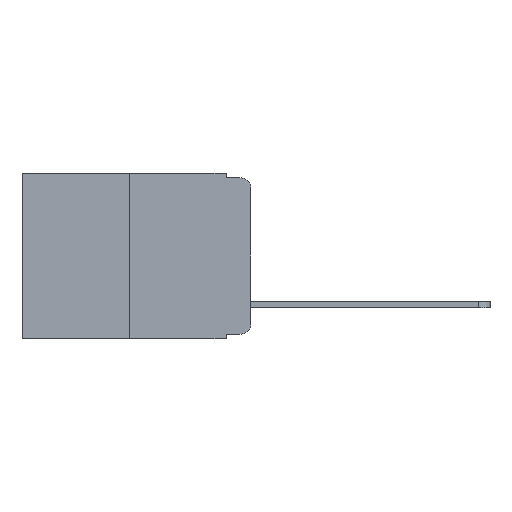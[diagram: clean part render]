
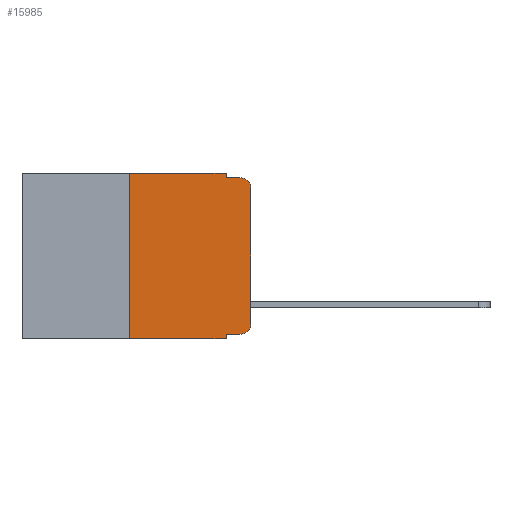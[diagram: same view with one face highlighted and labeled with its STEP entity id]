
A CAD part, left-side view. The second image highlights one B-rep face of the part: STEP entity #15985.
In plain terms, the highlighted planar face has unit normal (-1, 0, 0).
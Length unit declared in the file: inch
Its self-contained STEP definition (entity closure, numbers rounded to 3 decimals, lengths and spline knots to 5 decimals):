
#923 = VERTEX_POINT ( 'NONE', #13143 ) ;
#1006 = VERTEX_POINT ( 'NONE', #2256 ) ;
#1129 = CARTESIAN_POINT ( 'NONE',  ( 0., 0., 0. ) ) ;
#1184 = DIRECTION ( 'NONE',  ( 1., 0., 0. ) ) ;
#1445 = AXIS2_PLACEMENT_3D ( 'NONE', #12316, #3045, #13771 ) ;
#1646 = CARTESIAN_POINT ( 'NONE',  ( 0., 0.02, -0.01 ) ) ;
#1650 = CARTESIAN_POINT ( 'NONE',  ( 0., 0.051, -0.343 ) ) ;
#1653 = CIRCLE ( 'NONE', #1445, 0.02 ) ;
#1670 = CARTESIAN_POINT ( 'NONE',  ( 0., 0.473, -0.343 ) ) ;
#1677 = VERTEX_POINT ( 'NONE', #1650 ) ;
#2256 = CARTESIAN_POINT ( 'NONE',  ( 0., 0., -0.03 ) ) ;
#2742 = CARTESIAN_POINT ( 'NONE',  ( 0., 0.25, 0. ) ) ;
#2957 = LINE ( 'NONE', #1670, #15027 ) ;
#3012 = CARTESIAN_POINT ( 'NONE',  ( 0., 0.051, -0.01 ) ) ;
#3045 = DIRECTION ( 'NONE',  ( -1., 0., 0. ) ) ;
#3402 = DIRECTION ( 'NONE',  ( 0., -1., 0. ) ) ;
#3897 = VECTOR ( 'NONE', #16217, 39.37008 ) ;
#4248 = ORIENTED_EDGE ( 'NONE', *, *, #9250, .F. ) ;
#4501 = VECTOR ( 'NONE', #13741, 39.37008 ) ;
#4790 = ORIENTED_EDGE ( 'NONE', *, *, #9302, .F. ) ;
#4980 = DIRECTION ( 'NONE',  ( 0., 0., -1. ) ) ;
#5019 = CIRCLE ( 'NONE', #13310, 0.02 ) ;
#5287 = ORIENTED_EDGE ( 'NONE', *, *, #7506, .T. ) ;
#5894 = EDGE_CURVE ( 'NONE', #7233, #923, #14680, .T. ) ;
#5924 = CARTESIAN_POINT ( 'NONE',  ( 0., 0.051, -0.01 ) ) ;
#6185 = CARTESIAN_POINT ( 'NONE',  ( 0., 0.25, 0. ) ) ;
#6315 = CARTESIAN_POINT ( 'NONE',  ( 0., 0.051, -0.333 ) ) ;
#6357 = CARTESIAN_POINT ( 'NONE',  ( 0., 0.02, -0.03 ) ) ;
#6660 = VERTEX_POINT ( 'NONE', #11933 ) ;
#6905 = VECTOR ( 'NONE', #14562, 39.37008 ) ;
#7233 = VERTEX_POINT ( 'NONE', #2742 ) ;
#7506 = EDGE_CURVE ( 'NONE', #13405, #1677, #2957, .T. ) ;
#7651 = VECTOR ( 'NONE', #4980, 39.37008 ) ;
#7692 = CARTESIAN_POINT ( 'NONE',  ( 0., 0.051, 0. ) ) ;
#7870 = DIRECTION ( 'NONE',  ( 0., 0., -1. ) ) ;
#8481 = AXIS2_PLACEMENT_3D ( 'NONE', #9200, #1184, #12219 ) ;
#8831 = ORIENTED_EDGE ( 'NONE', *, *, #5894, .F. ) ;
#9151 = DIRECTION ( 'NONE',  ( 0., 0., 1. ) ) ;
#9200 = CARTESIAN_POINT ( 'NONE',  ( 0., 0.473, 0. ) ) ;
#9202 = EDGE_CURVE ( 'NONE', #10691, #1006, #17277, .T. ) ;
#9249 = EDGE_CURVE ( 'NONE', #1006, #10289, #5019, .T. ) ;
#9250 = EDGE_CURVE ( 'NONE', #18162, #10289, #16505, .T. ) ;
#9281 = ORIENTED_EDGE ( 'NONE', *, *, #10593, .F. ) ;
#9302 = EDGE_CURVE ( 'NONE', #923, #18162, #18215, .T. ) ;
#10289 = VERTEX_POINT ( 'NONE', #1646 ) ;
#10583 = EDGE_CURVE ( 'NONE', #13405, #7233, #18950, .T. ) ;
#10593 = EDGE_CURVE ( 'NONE', #14069, #1677, #18170, .T. ) ;
#10640 = EDGE_CURVE ( 'NONE', #14069, #6660, #17005, .T. ) ;
#10641 = EDGE_CURVE ( 'NONE', #6660, #10691, #1653, .T. ) ;
#10691 = VERTEX_POINT ( 'NONE', #12448 ) ;
#11402 = ORIENTED_EDGE ( 'NONE', *, *, #9202, .T. ) ;
#11933 = CARTESIAN_POINT ( 'NONE',  ( 0., 0.02, -0.333 ) ) ;
#12219 = DIRECTION ( 'NONE',  ( 0., 0., -1. ) ) ;
#12316 = CARTESIAN_POINT ( 'NONE',  ( 0., 0.02, -0.313 ) ) ;
#12448 = CARTESIAN_POINT ( 'NONE',  ( 0., 0., -0.313 ) ) ;
#12775 = ORIENTED_EDGE ( 'NONE', *, *, #10583, .F. ) ;
#13143 = CARTESIAN_POINT ( 'NONE',  ( 0., 0.051, 0. ) ) ;
#13244 = ORIENTED_EDGE ( 'NONE', *, *, #10640, .T. ) ;
#13310 = AXIS2_PLACEMENT_3D ( 'NONE', #6357, #16346, #7870 ) ;
#13405 = VERTEX_POINT ( 'NONE', #16231 ) ;
#13569 = VECTOR ( 'NONE', #17552, 39.37008 ) ;
#13741 = DIRECTION ( 'NONE',  ( 0., -1., 0. ) ) ;
#13771 = DIRECTION ( 'NONE',  ( 0., 0., -1. ) ) ;
#13917 = CARTESIAN_POINT ( 'NONE',  ( 0., 0.051, 0. ) ) ;
#14069 = VERTEX_POINT ( 'NONE', #15320 ) ;
#14320 = VECTOR ( 'NONE', #9151, 39.37008 ) ;
#14562 = DIRECTION ( 'NONE',  ( 0., -1., 0. ) ) ;
#14680 = LINE ( 'NONE', #17100, #6905 ) ;
#14898 = VECTOR ( 'NONE', #15004, 39.37008 ) ;
#15004 = DIRECTION ( 'NONE',  ( 0., 0., -1. ) ) ;
#15027 = VECTOR ( 'NONE', #3402, 39.37008 ) ;
#15151 = ORIENTED_EDGE ( 'NONE', *, *, #9249, .T. ) ;
#15320 = CARTESIAN_POINT ( 'NONE',  ( 0., 0.051, -0.333 ) ) ;
#15985 = ADVANCED_FACE ( 'NONE', ( #16322 ), #18679, .F. ) ;
#16217 = DIRECTION ( 'NONE',  ( 0., 0., 1. ) ) ;
#16231 = CARTESIAN_POINT ( 'NONE',  ( 0., 0.25, -0.343 ) ) ;
#16322 = FACE_OUTER_BOUND ( 'NONE', #18173, .T. ) ;
#16346 = DIRECTION ( 'NONE',  ( -1., 0., 0. ) ) ;
#16505 = LINE ( 'NONE', #3012, #4501 ) ;
#16723 = ORIENTED_EDGE ( 'NONE', *, *, #10641, .T. ) ;
#17005 = LINE ( 'NONE', #6315, #13569 ) ;
#17100 = CARTESIAN_POINT ( 'NONE',  ( 0., 0.473, 0. ) ) ;
#17277 = LINE ( 'NONE', #1129, #14320 ) ;
#17552 = DIRECTION ( 'NONE',  ( 0., -1., 0. ) ) ;
#18162 = VERTEX_POINT ( 'NONE', #5924 ) ;
#18170 = LINE ( 'NONE', #7692, #14898 ) ;
#18173 = EDGE_LOOP ( 'NONE', ( #11402, #15151, #4248, #4790, #8831, #12775, #5287, #9281, #13244, #16723 ) ) ;
#18215 = LINE ( 'NONE', #13917, #7651 ) ;
#18679 = PLANE ( 'NONE',  #8481 ) ;
#18950 = LINE ( 'NONE', #6185, #3897 ) ;
